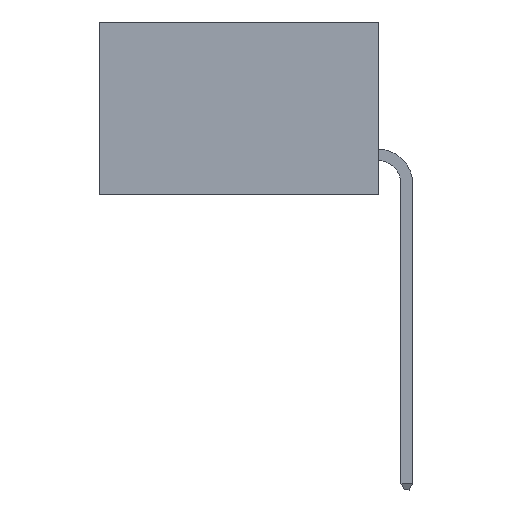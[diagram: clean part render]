
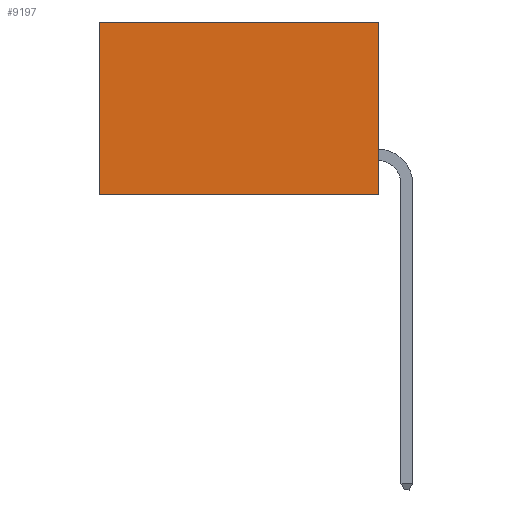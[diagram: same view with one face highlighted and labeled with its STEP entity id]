
A CAD part, left-side view. The second image highlights one B-rep face of the part: STEP entity #9197.
In plain terms, the highlighted planar face has unit normal (-1, 0, 0).
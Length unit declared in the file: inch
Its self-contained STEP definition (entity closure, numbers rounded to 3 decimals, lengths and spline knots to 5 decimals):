
#624 = ORIENTED_EDGE ( 'NONE', *, *, #11500, .F. ) ;
#724 = DIRECTION ( 'NONE',  ( 1., 0., 0. ) ) ;
#1077 = EDGE_CURVE ( 'NONE', #10716, #5736, #2855, .T. ) ;
#1867 = VECTOR ( 'NONE', #10637, 39.37008 ) ;
#2624 = CARTESIAN_POINT ( 'NONE',  ( 0.2615, 0., -0.37 ) ) ;
#2791 = CARTESIAN_POINT ( 'NONE',  ( 0.2615, 0., 0. ) ) ;
#2855 = LINE ( 'NONE', #8829, #5573 ) ;
#3571 = DIRECTION ( 'NONE',  ( 0., 0., -1. ) ) ;
#4426 = CARTESIAN_POINT ( 'NONE',  ( 0.2615, 0., -0.37 ) ) ;
#4496 = ORIENTED_EDGE ( 'NONE', *, *, #1077, .F. ) ;
#4606 = EDGE_CURVE ( 'NONE', #11608, #11182, #7965, .T. ) ;
#5133 = ORIENTED_EDGE ( 'NONE', *, *, #8636, .T. ) ;
#5268 = PLANE ( 'NONE',  #5412 ) ;
#5412 = AXIS2_PLACEMENT_3D ( 'NONE', #2624, #724, #3571 ) ;
#5572 = ORIENTED_EDGE ( 'NONE', *, *, #4606, .T. ) ;
#5573 = VECTOR ( 'NONE', #11770, 39.37008 ) ;
#5736 = VERTEX_POINT ( 'NONE', #4426 ) ;
#6508 = CARTESIAN_POINT ( 'NONE',  ( 0.2615, 0., -0.37 ) ) ;
#6963 = CARTESIAN_POINT ( 'NONE',  ( 0.2615, 0.6, -0.37 ) ) ;
#7965 = LINE ( 'NONE', #10768, #1867 ) ;
#8636 = EDGE_CURVE ( 'NONE', #10716, #11608, #9946, .T. ) ;
#8829 = CARTESIAN_POINT ( 'NONE',  ( 0.2615, 0., -0.37 ) ) ;
#9197 = ADVANCED_FACE ( 'NONE', ( #12230 ), #5268, .F. ) ;
#9946 = LINE ( 'NONE', #10002, #10644 ) ;
#10002 = CARTESIAN_POINT ( 'NONE',  ( 0.2615, 0., 0. ) ) ;
#10484 = VECTOR ( 'NONE', #11461, 39.37008 ) ;
#10637 = DIRECTION ( 'NONE',  ( 0., 0., -1. ) ) ;
#10644 = VECTOR ( 'NONE', #11995, 39.37008 ) ;
#10716 = VERTEX_POINT ( 'NONE', #2791 ) ;
#10768 = CARTESIAN_POINT ( 'NONE',  ( 0.2615, 0.6, -0.37 ) ) ;
#10820 = CARTESIAN_POINT ( 'NONE',  ( 0.2615, 0.6, 0. ) ) ;
#10869 = EDGE_LOOP ( 'NONE', ( #5572, #624, #4496, #5133 ) ) ;
#11182 = VERTEX_POINT ( 'NONE', #6963 ) ;
#11461 = DIRECTION ( 'NONE',  ( 0., 1., 0. ) ) ;
#11500 = EDGE_CURVE ( 'NONE', #5736, #11182, #11527, .T. ) ;
#11527 = LINE ( 'NONE', #6508, #10484 ) ;
#11608 = VERTEX_POINT ( 'NONE', #10820 ) ;
#11770 = DIRECTION ( 'NONE',  ( 0., 0., -1. ) ) ;
#11995 = DIRECTION ( 'NONE',  ( 0., 1., 0. ) ) ;
#12230 = FACE_OUTER_BOUND ( 'NONE', #10869, .T. ) ;
